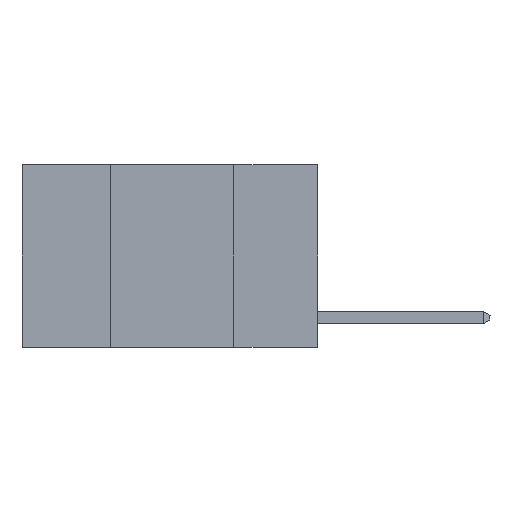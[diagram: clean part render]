
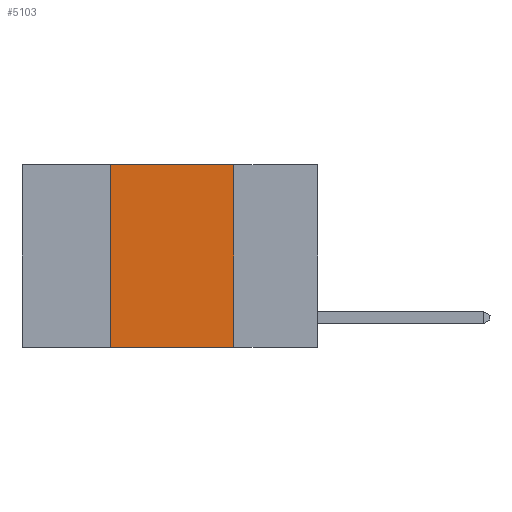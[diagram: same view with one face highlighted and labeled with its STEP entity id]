
A CAD part, left-side view. The second image highlights one B-rep face of the part: STEP entity #5103.
In plain terms, the highlighted planar face has unit normal (-1, 0, 0).
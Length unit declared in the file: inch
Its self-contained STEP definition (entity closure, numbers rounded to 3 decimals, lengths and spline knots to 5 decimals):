
#77 = VERTEX_POINT ( 'NONE', #10181 ) ;
#458 = ORIENTED_EDGE ( 'NONE', *, *, #9336, .T. ) ;
#1145 = EDGE_CURVE ( 'NONE', #8858, #77, #7864, .T. ) ;
#1739 = DIRECTION ( 'NONE',  ( 1., 0., 0. ) ) ;
#2106 = VERTEX_POINT ( 'NONE', #8857 ) ;
#2808 = LINE ( 'NONE', #8099, #8035 ) ;
#3734 = DIRECTION ( 'NONE',  ( 0., -1., 0. ) ) ;
#3982 = AXIS2_PLACEMENT_3D ( 'NONE', #10069, #1739, #13210 ) ;
#4506 = VERTEX_POINT ( 'NONE', #9820 ) ;
#4836 = LINE ( 'NONE', #10559, #9699 ) ;
#5103 = ADVANCED_FACE ( 'NONE', ( #6933 ), #12319, .F. ) ;
#5834 = CARTESIAN_POINT ( 'NONE',  ( 0., 0.6, 0. ) ) ;
#5930 = DIRECTION ( 'NONE',  ( 0., -1., 0. ) ) ;
#5958 = EDGE_LOOP ( 'NONE', ( #6362, #6724, #10329, #458 ) ) ;
#6250 = DIRECTION ( 'NONE',  ( 0., 0., -1. ) ) ;
#6362 = ORIENTED_EDGE ( 'NONE', *, *, #6542, .F. ) ;
#6542 = EDGE_CURVE ( 'NONE', #77, #2106, #4836, .T. ) ;
#6724 = ORIENTED_EDGE ( 'NONE', *, *, #1145, .F. ) ;
#6933 = FACE_OUTER_BOUND ( 'NONE', #5958, .T. ) ;
#7252 = VECTOR ( 'NONE', #3734, 39.37008 ) ;
#7622 = DIRECTION ( 'NONE',  ( 0., 0., 1. ) ) ;
#7685 = LINE ( 'NONE', #7760, #11814 ) ;
#7760 = CARTESIAN_POINT ( 'NONE',  ( 0., 0.42, 0. ) ) ;
#7864 = LINE ( 'NONE', #5834, #7252 ) ;
#8028 = EDGE_CURVE ( 'NONE', #4506, #8858, #7685, .T. ) ;
#8035 = VECTOR ( 'NONE', #5930, 39.37008 ) ;
#8099 = CARTESIAN_POINT ( 'NONE',  ( 0., 0.6, -0.37 ) ) ;
#8857 = CARTESIAN_POINT ( 'NONE',  ( 0., 0.17, -0.37 ) ) ;
#8858 = VERTEX_POINT ( 'NONE', #8893 ) ;
#8893 = CARTESIAN_POINT ( 'NONE',  ( 0., 0.42, 0. ) ) ;
#9336 = EDGE_CURVE ( 'NONE', #4506, #2106, #2808, .T. ) ;
#9699 = VECTOR ( 'NONE', #6250, 39.37008 ) ;
#9820 = CARTESIAN_POINT ( 'NONE',  ( 0., 0.42, -0.37 ) ) ;
#10069 = CARTESIAN_POINT ( 'NONE',  ( 0., 0.6, 0. ) ) ;
#10181 = CARTESIAN_POINT ( 'NONE',  ( 0., 0.17, 0. ) ) ;
#10329 = ORIENTED_EDGE ( 'NONE', *, *, #8028, .F. ) ;
#10559 = CARTESIAN_POINT ( 'NONE',  ( 0., 0.17, 0. ) ) ;
#11814 = VECTOR ( 'NONE', #7622, 39.37008 ) ;
#12319 = PLANE ( 'NONE',  #3982 ) ;
#13210 = DIRECTION ( 'NONE',  ( 0., 0., -1. ) ) ;
